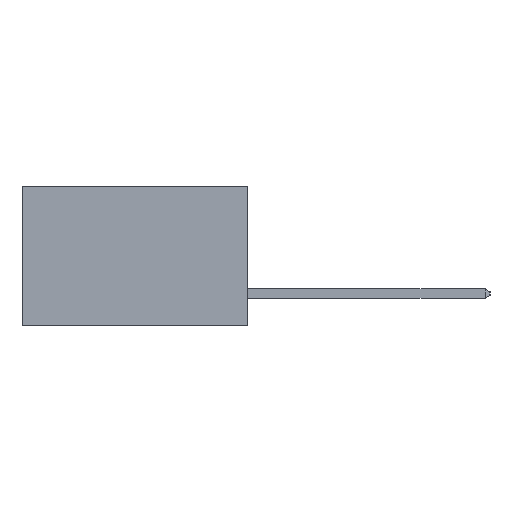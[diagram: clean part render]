
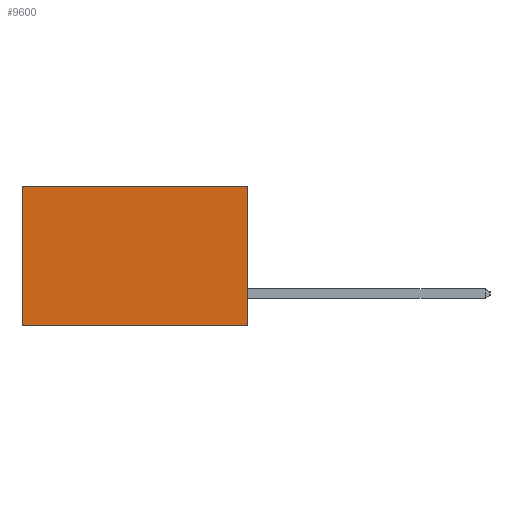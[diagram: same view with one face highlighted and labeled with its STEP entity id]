
A CAD part, left-side view. The second image highlights one B-rep face of the part: STEP entity #9600.
In plain terms, the highlighted planar face has unit normal (-1, 0, 0).
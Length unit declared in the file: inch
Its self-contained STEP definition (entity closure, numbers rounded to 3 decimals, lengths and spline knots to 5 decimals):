
#212 = VECTOR ( 'NONE', #5543, 39.37008 ) ;
#1029 = ORIENTED_EDGE ( 'NONE', *, *, #7371, .F. ) ;
#1443 = DIRECTION ( 'NONE',  ( 0., 0., -1. ) ) ;
#1494 = CARTESIAN_POINT ( 'NONE',  ( 0.298, 0.6, 0. ) ) ;
#1575 = AXIS2_PLACEMENT_3D ( 'NONE', #8170, #4172, #9737 ) ;
#1927 = FACE_OUTER_BOUND ( 'NONE', #10337, .T. ) ;
#2029 = LINE ( 'NONE', #1494, #6219 ) ;
#2097 = DIRECTION ( 'NONE',  ( 0., 0., -1. ) ) ;
#2417 = VECTOR ( 'NONE', #4630, 39.37008 ) ;
#2570 = LINE ( 'NONE', #2997, #212 ) ;
#2665 = VERTEX_POINT ( 'NONE', #10432 ) ;
#2997 = CARTESIAN_POINT ( 'NONE',  ( 0.298, 0., -0.37 ) ) ;
#3157 = CARTESIAN_POINT ( 'NONE',  ( 0.298, 0., -0.37 ) ) ;
#3288 = PLANE ( 'NONE',  #1575 ) ;
#3403 = EDGE_CURVE ( 'NONE', #9405, #2665, #2029, .T. ) ;
#3451 = VECTOR ( 'NONE', #2097, 39.37008 ) ;
#3578 = EDGE_CURVE ( 'NONE', #9574, #9405, #7101, .T. ) ;
#4172 = DIRECTION ( 'NONE',  ( 1., 0., 0. ) ) ;
#4630 = DIRECTION ( 'NONE',  ( 0., 1., 0. ) ) ;
#4744 = CARTESIAN_POINT ( 'NONE',  ( 0.298, 0.6, 0. ) ) ;
#5543 = DIRECTION ( 'NONE',  ( 0., 1., 0. ) ) ;
#5553 = CARTESIAN_POINT ( 'NONE',  ( 0.298, 0., 0. ) ) ;
#5721 = CARTESIAN_POINT ( 'NONE',  ( 0.298, 0., 0. ) ) ;
#5762 = ORIENTED_EDGE ( 'NONE', *, *, #3403, .T. ) ;
#6219 = VECTOR ( 'NONE', #1443, 39.37008 ) ;
#7101 = LINE ( 'NONE', #7328, #2417 ) ;
#7328 = CARTESIAN_POINT ( 'NONE',  ( 0.298, 0., 0. ) ) ;
#7371 = EDGE_CURVE ( 'NONE', #9574, #7671, #10084, .T. ) ;
#7671 = VERTEX_POINT ( 'NONE', #3157 ) ;
#8170 = CARTESIAN_POINT ( 'NONE',  ( 0.298, 0., 0. ) ) ;
#8232 = EDGE_CURVE ( 'NONE', #7671, #2665, #2570, .T. ) ;
#8287 = ORIENTED_EDGE ( 'NONE', *, *, #3578, .T. ) ;
#9405 = VERTEX_POINT ( 'NONE', #4744 ) ;
#9574 = VERTEX_POINT ( 'NONE', #5721 ) ;
#9600 = ADVANCED_FACE ( 'NONE', ( #1927 ), #3288, .F. ) ;
#9737 = DIRECTION ( 'NONE',  ( 0., 0., -1. ) ) ;
#10084 = LINE ( 'NONE', #5553, #3451 ) ;
#10095 = ORIENTED_EDGE ( 'NONE', *, *, #8232, .F. ) ;
#10337 = EDGE_LOOP ( 'NONE', ( #5762, #10095, #1029, #8287 ) ) ;
#10432 = CARTESIAN_POINT ( 'NONE',  ( 0.298, 0.6, -0.37 ) ) ;
